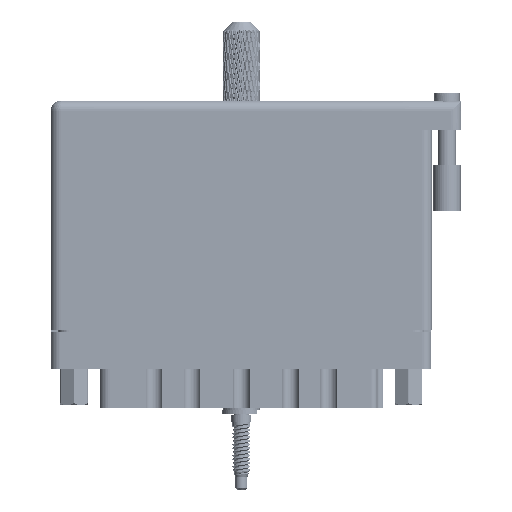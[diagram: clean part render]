
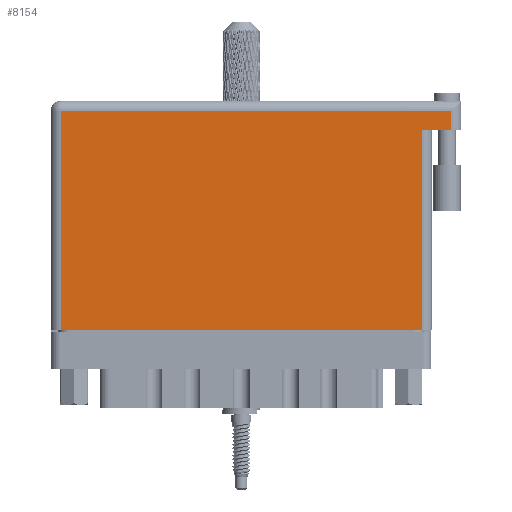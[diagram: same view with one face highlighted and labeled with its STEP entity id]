
A CAD part, front view. The second image highlights one B-rep face of the part: STEP entity #8154.
In plain terms, the highlighted face is planar.
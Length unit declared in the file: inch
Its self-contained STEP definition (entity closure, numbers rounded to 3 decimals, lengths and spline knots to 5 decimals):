
#2330 = LINE ( 'NONE', #90824, #85505 ) ;
#2563 = VERTEX_POINT ( 'NONE', #13392 ) ;
#2809 = LINE ( 'NONE', #32552, #94378 ) ;
#6487 = EDGE_CURVE ( 'NONE', #24242, #19413, #91243, .T. ) ;
#6566 = ORIENTED_EDGE ( 'NONE', *, *, #6487, .T. ) ;
#8154 = ADVANCED_FACE ( 'NONE', ( #87207 ), #25887, .F. ) ;
#9815 = CARTESIAN_POINT ( 'NONE',  ( 2.73, 1.369, 0. ) ) ;
#12075 = VECTOR ( 'NONE', #30667, 39.37008 ) ;
#13392 = CARTESIAN_POINT ( 'NONE',  ( 0.07, 0., 0. ) ) ;
#13980 = EDGE_CURVE ( 'NONE', #31999, #92023, #39135, .T. ) ;
#15340 = DIRECTION ( 'NONE',  ( 0., -1., 0. ) ) ;
#19413 = VERTEX_POINT ( 'NONE', #88332 ) ;
#23320 = VECTOR ( 'NONE', #15340, 39.37008 ) ;
#24242 = VERTEX_POINT ( 'NONE', #74030 ) ;
#25887 = PLANE ( 'NONE',  #51787 ) ;
#27242 = VECTOR ( 'NONE', #90371, 39.37008 ) ;
#30257 = ORIENTED_EDGE ( 'NONE', *, *, #46522, .T. ) ;
#30667 = DIRECTION ( 'NONE',  ( 0., 1., 0. ) ) ;
#31999 = VERTEX_POINT ( 'NONE', #9815 ) ;
#32552 = CARTESIAN_POINT ( 'NONE',  ( 2.8, 1.369, 0. ) ) ;
#32704 = DIRECTION ( 'NONE',  ( -1., 0., 0. ) ) ;
#34972 = DIRECTION ( 'NONE',  ( 0., 0., -1. ) ) ;
#39135 = LINE ( 'NONE', #86920, #12075 ) ;
#43162 = LINE ( 'NONE', #52184, #23320 ) ;
#46522 = EDGE_CURVE ( 'NONE', #2563, #24242, #52906, .T. ) ;
#51787 = AXIS2_PLACEMENT_3D ( 'NONE', #56888, #34972, #64629 ) ;
#52184 = CARTESIAN_POINT ( 'NONE',  ( 0.07, 0., 0. ) ) ;
#52906 = LINE ( 'NONE', #81956, #27242 ) ;
#53941 = ORIENTED_EDGE ( 'NONE', *, *, #13980, .T. ) ;
#55987 = CARTESIAN_POINT ( 'NONE',  ( 2.73, 1.496, 0. ) ) ;
#56888 = CARTESIAN_POINT ( 'NONE',  ( 0., 1.566, 0. ) ) ;
#56909 = EDGE_CURVE ( 'NONE', #92023, #80257, #2330, .T. ) ;
#59968 = ORIENTED_EDGE ( 'NONE', *, *, #106541, .F. ) ;
#64253 = EDGE_LOOP ( 'NONE', ( #30257, #6566, #59968, #53941, #91266, #91521 ) ) ;
#64629 = DIRECTION ( 'NONE',  ( -1., 0., 0. ) ) ;
#69273 = CARTESIAN_POINT ( 'NONE',  ( 0.07, 1.496, 0. ) ) ;
#71918 = DIRECTION ( 'NONE',  ( -1., 0., 0. ) ) ;
#71923 = VECTOR ( 'NONE', #99675, 39.37008 ) ;
#74030 = CARTESIAN_POINT ( 'NONE',  ( 2.53, 0., 0. ) ) ;
#79645 = CARTESIAN_POINT ( 'NONE',  ( 2.53, 1.369, 0. ) ) ;
#80257 = VERTEX_POINT ( 'NONE', #69273 ) ;
#81956 = CARTESIAN_POINT ( 'NONE',  ( 0., 0., 0. ) ) ;
#85468 = EDGE_CURVE ( 'NONE', #80257, #2563, #43162, .T. ) ;
#85505 = VECTOR ( 'NONE', #32704, 39.37008 ) ;
#86920 = CARTESIAN_POINT ( 'NONE',  ( 2.73, 1.566, 0. ) ) ;
#87207 = FACE_OUTER_BOUND ( 'NONE', #64253, .T. ) ;
#88332 = CARTESIAN_POINT ( 'NONE',  ( 2.53, 1.369, 0. ) ) ;
#90371 = DIRECTION ( 'NONE',  ( 1., 0., 0. ) ) ;
#90824 = CARTESIAN_POINT ( 'NONE',  ( 0., 1.496, 0. ) ) ;
#91243 = LINE ( 'NONE', #79645, #71923 ) ;
#91266 = ORIENTED_EDGE ( 'NONE', *, *, #56909, .T. ) ;
#91521 = ORIENTED_EDGE ( 'NONE', *, *, #85468, .T. ) ;
#92023 = VERTEX_POINT ( 'NONE', #55987 ) ;
#94378 = VECTOR ( 'NONE', #71918, 39.37008 ) ;
#99675 = DIRECTION ( 'NONE',  ( 0., 1., 0. ) ) ;
#106541 = EDGE_CURVE ( 'NONE', #31999, #19413, #2809, .T. ) ;
